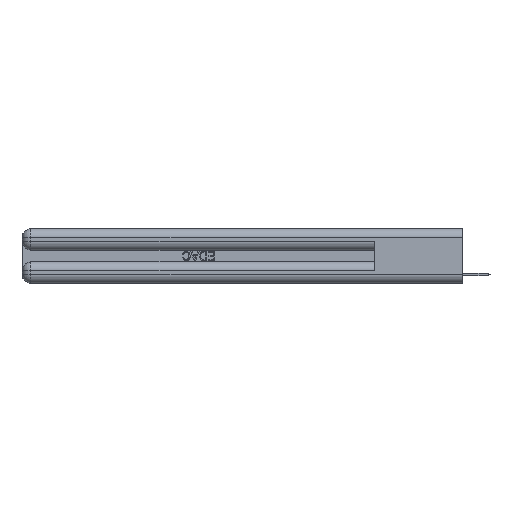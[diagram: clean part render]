
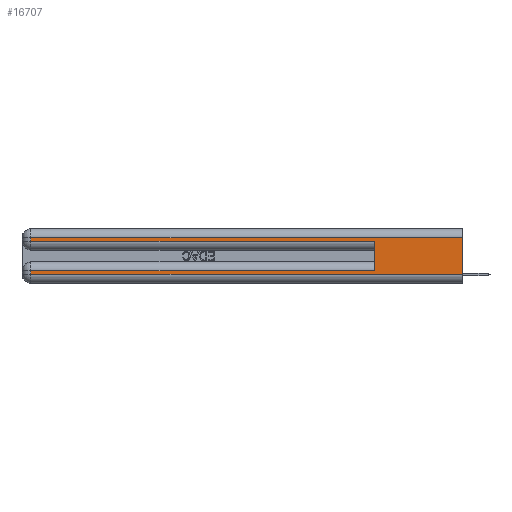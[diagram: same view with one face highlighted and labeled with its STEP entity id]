
A CAD part, left-side view. The second image highlights one B-rep face of the part: STEP entity #16707.
In plain terms, the highlighted planar face has unit normal (-1, 0, 0).
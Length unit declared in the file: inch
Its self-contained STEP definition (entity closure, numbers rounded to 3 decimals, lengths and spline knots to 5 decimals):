
#615 = CARTESIAN_POINT ( 'NONE',  ( 0., 0., 0.085 ) ) ;
#1078 = CARTESIAN_POINT ( 'NONE',  ( 0., 0., 0.06 ) ) ;
#1118 = ORIENTED_EDGE ( 'NONE', *, *, #8960, .T. ) ;
#2268 = VERTEX_POINT ( 'NONE', #20680 ) ;
#2339 = EDGE_CURVE ( 'NONE', #30043, #27613, #17417, .T. ) ;
#2912 = VECTOR ( 'NONE', #12638, 39.37008 ) ;
#2968 = CARTESIAN_POINT ( 'NONE',  ( 0., 0., 0.31 ) ) ;
#3165 = CARTESIAN_POINT ( 'NONE',  ( 0., 2.94, 0.31 ) ) ;
#4071 = LINE ( 'NONE', #17379, #14776 ) ;
#4375 = VECTOR ( 'NONE', #28010, 39.37008 ) ;
#4575 = CARTESIAN_POINT ( 'NONE',  ( 0., 0., 0.06 ) ) ;
#7009 = DIRECTION ( 'NONE',  ( 0., 0., 1. ) ) ;
#7019 = CARTESIAN_POINT ( 'NONE',  ( 0., 0., 0.37 ) ) ;
#7276 = AXIS2_PLACEMENT_3D ( 'NONE', #7019, #31659, #14240 ) ;
#7299 = ORIENTED_EDGE ( 'NONE', *, *, #12808, .T. ) ;
#7425 = EDGE_CURVE ( 'NONE', #30007, #27122, #4071, .T. ) ;
#8320 = CARTESIAN_POINT ( 'NONE',  ( 0., 0.6, 0.085 ) ) ;
#8960 = EDGE_CURVE ( 'NONE', #12491, #2268, #14435, .T. ) ;
#9077 = VECTOR ( 'NONE', #15466, 39.37008 ) ;
#9178 = CARTESIAN_POINT ( 'NONE',  ( 0., 2.94, 0.37 ) ) ;
#10333 = LINE ( 'NONE', #29884, #28439 ) ;
#10386 = VERTEX_POINT ( 'NONE', #3165 ) ;
#10892 = ORIENTED_EDGE ( 'NONE', *, *, #25085, .T. ) ;
#12491 = VERTEX_POINT ( 'NONE', #24305 ) ;
#12638 = DIRECTION ( 'NONE',  ( 0., 0., -1. ) ) ;
#12808 = EDGE_CURVE ( 'NONE', #30007, #10386, #10333, .T. ) ;
#12895 = FACE_OUTER_BOUND ( 'NONE', #27498, .T. ) ;
#13205 = CARTESIAN_POINT ( 'NONE',  ( 0., 0.6, 0.285 ) ) ;
#13658 = ORIENTED_EDGE ( 'NONE', *, *, #16584, .T. ) ;
#14240 = DIRECTION ( 'NONE',  ( 0., 0., -1. ) ) ;
#14435 = LINE ( 'NONE', #22767, #2912 ) ;
#14776 = VECTOR ( 'NONE', #29547, 39.37008 ) ;
#14920 = DIRECTION ( 'NONE',  ( 0., -1., 0. ) ) ;
#15210 = CARTESIAN_POINT ( 'NONE',  ( 0., 2.94, 0.285 ) ) ;
#15466 = DIRECTION ( 'NONE',  ( 0., 1., 0. ) ) ;
#15627 = LINE ( 'NONE', #615, #9077 ) ;
#16294 = LINE ( 'NONE', #9178, #4375 ) ;
#16497 = DIRECTION ( 'NONE',  ( 0., -1., 0. ) ) ;
#16584 = EDGE_CURVE ( 'NONE', #30043, #12491, #15627, .T. ) ;
#16707 = ADVANCED_FACE ( 'NONE', ( #12895 ), #21761, .F. ) ;
#16910 = CARTESIAN_POINT ( 'NONE',  ( 0., 0.6, 0.145 ) ) ;
#17379 = CARTESIAN_POINT ( 'NONE',  ( 0., 0., 0.37 ) ) ;
#17417 = LINE ( 'NONE', #16910, #31649 ) ;
#18956 = LINE ( 'NONE', #29689, #27828 ) ;
#20680 = CARTESIAN_POINT ( 'NONE',  ( 0., 2.94, 0.06 ) ) ;
#21621 = ORIENTED_EDGE ( 'NONE', *, *, #7425, .F. ) ;
#21761 = PLANE ( 'NONE',  #7276 ) ;
#22350 = EDGE_CURVE ( 'NONE', #24671, #27613, #18956, .T. ) ;
#22767 = CARTESIAN_POINT ( 'NONE',  ( 0., 2.94, 0.37 ) ) ;
#23569 = ORIENTED_EDGE ( 'NONE', *, *, #30249, .T. ) ;
#24305 = CARTESIAN_POINT ( 'NONE',  ( 0., 2.94, 0.085 ) ) ;
#24671 = VERTEX_POINT ( 'NONE', #15210 ) ;
#25042 = DIRECTION ( 'NONE',  ( 0., 1., 0. ) ) ;
#25085 = EDGE_CURVE ( 'NONE', #2268, #27122, #31844, .T. ) ;
#25175 = ORIENTED_EDGE ( 'NONE', *, *, #22350, .T. ) ;
#26396 = ORIENTED_EDGE ( 'NONE', *, *, #2339, .F. ) ;
#27122 = VERTEX_POINT ( 'NONE', #1078 ) ;
#27498 = EDGE_LOOP ( 'NONE', ( #21621, #7299, #23569, #25175, #26396, #13658, #1118, #10892 ) ) ;
#27613 = VERTEX_POINT ( 'NONE', #13205 ) ;
#27828 = VECTOR ( 'NONE', #14920, 39.37008 ) ;
#28010 = DIRECTION ( 'NONE',  ( 0., 0., -1. ) ) ;
#28439 = VECTOR ( 'NONE', #25042, 39.37008 ) ;
#29547 = DIRECTION ( 'NONE',  ( 0., 0., -1. ) ) ;
#29689 = CARTESIAN_POINT ( 'NONE',  ( 0., 0., 0.285 ) ) ;
#29884 = CARTESIAN_POINT ( 'NONE',  ( 0., 0., 0.31 ) ) ;
#30007 = VERTEX_POINT ( 'NONE', #2968 ) ;
#30043 = VERTEX_POINT ( 'NONE', #8320 ) ;
#30249 = EDGE_CURVE ( 'NONE', #10386, #24671, #16294, .T. ) ;
#30686 = VECTOR ( 'NONE', #16497, 39.37008 ) ;
#31649 = VECTOR ( 'NONE', #7009, 39.37008 ) ;
#31659 = DIRECTION ( 'NONE',  ( 1., 0., 0. ) ) ;
#31844 = LINE ( 'NONE', #4575, #30686 ) ;
